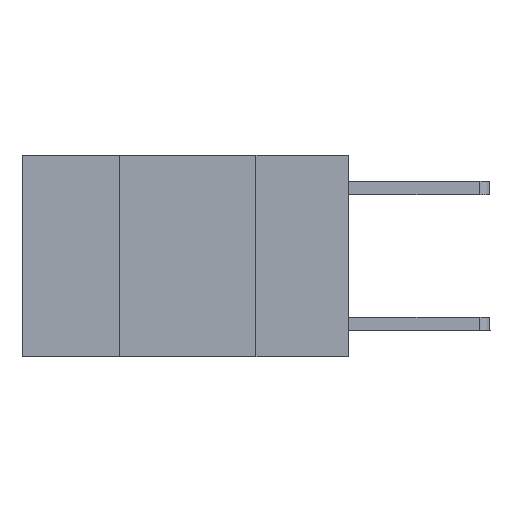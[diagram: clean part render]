
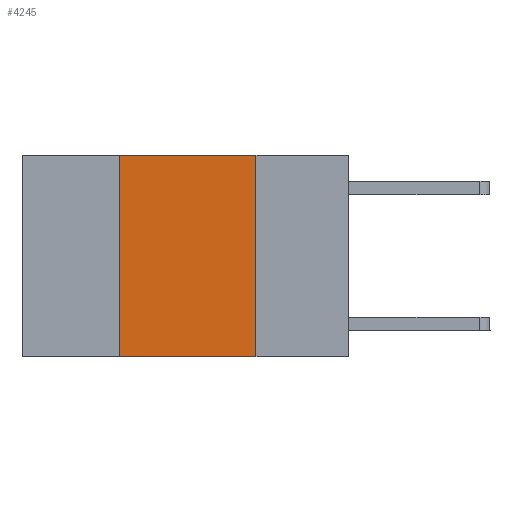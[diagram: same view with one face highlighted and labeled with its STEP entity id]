
A CAD part, left-side view. The second image highlights one B-rep face of the part: STEP entity #4245.
In plain terms, the highlighted planar face has unit normal (-1, 0, 0).
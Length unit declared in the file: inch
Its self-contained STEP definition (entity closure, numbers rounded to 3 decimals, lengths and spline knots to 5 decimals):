
#68 = CARTESIAN_POINT ( 'NONE',  ( 0., 0.6, -0.37 ) ) ;
#571 = PLANE ( 'NONE',  #10699 ) ;
#949 = DIRECTION ( 'NONE',  ( 0., -1., 0. ) ) ;
#1350 = ORIENTED_EDGE ( 'NONE', *, *, #7174, .F. ) ;
#1369 = CARTESIAN_POINT ( 'NONE',  ( 0., 0.6, 0. ) ) ;
#1384 = ORIENTED_EDGE ( 'NONE', *, *, #2693, .F. ) ;
#1533 = ORIENTED_EDGE ( 'NONE', *, *, #7032, .F. ) ;
#1720 = VECTOR ( 'NONE', #2655, 39.37008 ) ;
#1742 = CARTESIAN_POINT ( 'NONE',  ( 0., 0.17, 0. ) ) ;
#1764 = ORIENTED_EDGE ( 'NONE', *, *, #2364, .T. ) ;
#2031 = VECTOR ( 'NONE', #2231, 39.37008 ) ;
#2231 = DIRECTION ( 'NONE',  ( 0., -1., 0. ) ) ;
#2320 = VERTEX_POINT ( 'NONE', #3467 ) ;
#2364 = EDGE_CURVE ( 'NONE', #5030, #10375, #6486, .T. ) ;
#2385 = CARTESIAN_POINT ( 'NONE',  ( 0., 0.17, 0. ) ) ;
#2655 = DIRECTION ( 'NONE',  ( 0., 0., -1. ) ) ;
#2693 = EDGE_CURVE ( 'NONE', #2320, #8049, #5806, .T. ) ;
#3286 = DIRECTION ( 'NONE',  ( 0., 0., 1. ) ) ;
#3467 = CARTESIAN_POINT ( 'NONE',  ( 0., 0.42, 0. ) ) ;
#3605 = LINE ( 'NONE', #5860, #8180 ) ;
#4014 = LINE ( 'NONE', #1742, #1720 ) ;
#4245 = ADVANCED_FACE ( 'NONE', ( #5319 ), #571, .F. ) ;
#4924 = DIRECTION ( 'NONE',  ( 0., 0., -1. ) ) ;
#5030 = VERTEX_POINT ( 'NONE', #7873 ) ;
#5319 = FACE_OUTER_BOUND ( 'NONE', #8480, .T. ) ;
#5806 = LINE ( 'NONE', #1369, #2031 ) ;
#5860 = CARTESIAN_POINT ( 'NONE',  ( 0., 0.42, 0. ) ) ;
#6486 = LINE ( 'NONE', #68, #10317 ) ;
#7032 = EDGE_CURVE ( 'NONE', #5030, #2320, #3605, .T. ) ;
#7174 = EDGE_CURVE ( 'NONE', #8049, #10375, #4014, .T. ) ;
#7873 = CARTESIAN_POINT ( 'NONE',  ( 0., 0.42, -0.37 ) ) ;
#8049 = VERTEX_POINT ( 'NONE', #2385 ) ;
#8180 = VECTOR ( 'NONE', #3286, 39.37008 ) ;
#8308 = CARTESIAN_POINT ( 'NONE',  ( 0., 0.6, 0. ) ) ;
#8480 = EDGE_LOOP ( 'NONE', ( #1350, #1384, #1533, #1764 ) ) ;
#9883 = DIRECTION ( 'NONE',  ( 1., 0., 0. ) ) ;
#10317 = VECTOR ( 'NONE', #949, 39.37008 ) ;
#10375 = VERTEX_POINT ( 'NONE', #10529 ) ;
#10529 = CARTESIAN_POINT ( 'NONE',  ( 0., 0.17, -0.37 ) ) ;
#10699 = AXIS2_PLACEMENT_3D ( 'NONE', #8308, #9883, #4924 ) ;
